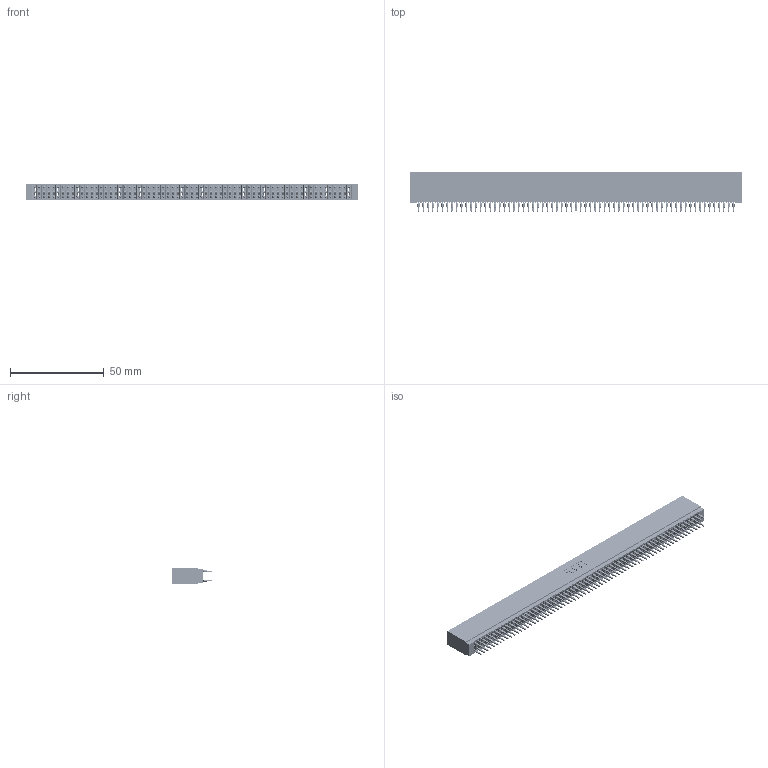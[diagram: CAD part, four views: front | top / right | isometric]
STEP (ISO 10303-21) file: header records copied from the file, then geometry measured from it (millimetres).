
FILE_DESCRIPTION (( 'STEP AP203' ), '1' );
FILE_NAME ('745-134-560-201.STEP', '2020-09-14T20:25:37', ( '' ), ( '' ), 'SwSTEP 2.0', 'SolidWorks 2020', '' );
FILE_SCHEMA (( 'CONFIG_CONTROL_DESIGN' ));
Length unit declared in the file: inch
Products named in the file (3): 745 Part_Insulator Option - 01; 745-134-560-201; 745-292-001_560
Assembly tree (135 placements, depth 2):
  745-134-560-201
    745 Part_Insulator Option - 01
    745-292-001_560  x134
Bounding box: 176.78 x 21.22 x 8.89 mm (x, y, z)
Volume: 16265.6 mm3; surface area: 35758.8 mm2
Topology: 135 solids, 135 shells, 13294 faces, 36371 edges, 23086 vertices
Faces by surface type: plane 6889, cylinder 2921, bspline 2680, torus 804
Entity records: 109712 total; most frequent: CARTESIAN_POINT 19525, ORIENTED_EDGE 19010, DIRECTION 16589, EDGE_CURVE 9505, LINE 8913, VECTOR 8913, VERTEX_POINT 6062, AXIS2_PLACEMENT_3D 3838
